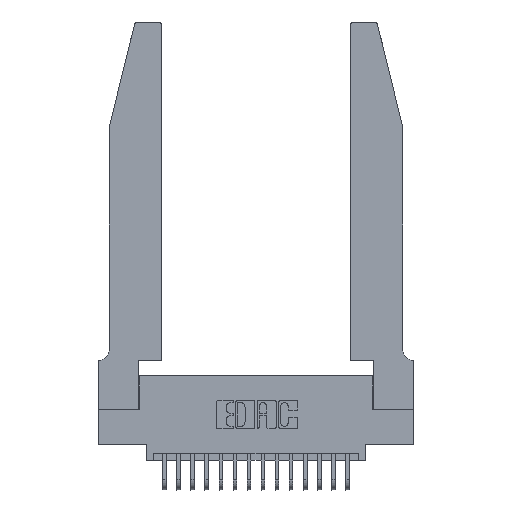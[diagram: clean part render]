
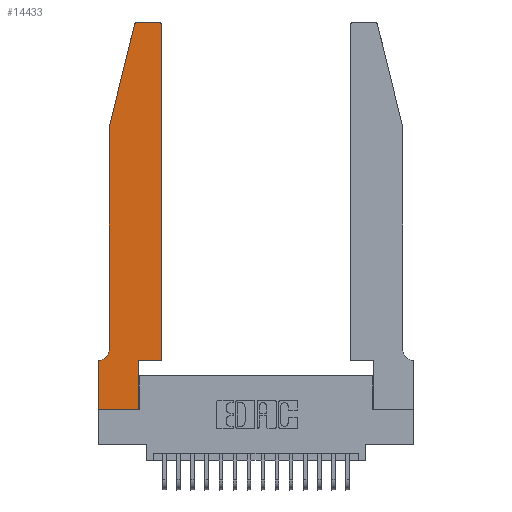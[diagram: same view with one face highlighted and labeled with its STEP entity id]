
A CAD part, top view. The second image highlights one B-rep face of the part: STEP entity #14433.
In plain terms, the highlighted planar face has unit normal (0, 0, 1).
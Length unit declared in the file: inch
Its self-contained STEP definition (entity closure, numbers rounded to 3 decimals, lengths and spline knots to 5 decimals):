
#6 = ORIENTED_EDGE ( 'NONE', *, *, #21173, .T. ) ;
#166 = VERTEX_POINT ( 'NONE', #15257 ) ;
#196 = EDGE_CURVE ( 'NONE', #13530, #4539, #17031, .T. ) ;
#664 = EDGE_CURVE ( 'NONE', #4786, #18224, #4362, .T. ) ;
#1320 = ORIENTED_EDGE ( 'NONE', *, *, #18303, .T. ) ;
#1442 = DIRECTION ( 'NONE',  ( 0., 1., 0. ) ) ;
#1481 = EDGE_CURVE ( 'NONE', #16555, #20800, #13324, .T. ) ;
#1889 = VERTEX_POINT ( 'NONE', #13498 ) ;
#1890 = LINE ( 'NONE', #8039, #14753 ) ;
#2274 = CARTESIAN_POINT ( 'NONE',  ( 0.0755, 2., 0.37 ) ) ;
#2402 = CARTESIAN_POINT ( 'NONE',  ( 0.4505, 0.35, 0.37 ) ) ;
#2846 = VECTOR ( 'NONE', #16586, 39.37008 ) ;
#3107 = AXIS2_PLACEMENT_3D ( 'NONE', #10799, #10655, #14158 ) ;
#3645 = CARTESIAN_POINT ( 'NONE',  ( 0.284, 2.72, 0.37 ) ) ;
#4362 = LINE ( 'NONE', #14949, #2846 ) ;
#4539 = VERTEX_POINT ( 'NONE', #11368 ) ;
#4607 = ORIENTED_EDGE ( 'NONE', *, *, #1481, .T. ) ;
#4786 = VERTEX_POINT ( 'NONE', #20607 ) ;
#4927 = CIRCLE ( 'NONE', #15768, 0.03 ) ;
#5079 = AXIS2_PLACEMENT_3D ( 'NONE', #3645, #16730, #18179 ) ;
#5161 = LINE ( 'NONE', #2402, #12854 ) ;
#5383 = DIRECTION ( 'NONE',  ( -1., 0., 0. ) ) ;
#5917 = EDGE_LOOP ( 'NONE', ( #13122, #15151, #10997, #10688, #4607, #13922, #11732, #10229, #1320, #17083, #6, #9298 ) ) ;
#5925 = CARTESIAN_POINT ( 'NONE',  ( 0.4505, 0.35, 0.37 ) ) ;
#6440 = VECTOR ( 'NONE', #19181, 39.37008 ) ;
#6522 = LINE ( 'NONE', #5925, #12433 ) ;
#6703 = VECTOR ( 'NONE', #5383, 39.37008 ) ;
#7192 = DIRECTION ( 'NONE',  ( 0., 1., 0. ) ) ;
#7670 = CARTESIAN_POINT ( 'NONE',  ( 0.4205, 2.75, 0.37 ) ) ;
#7751 = EDGE_CURVE ( 'NONE', #9254, #16555, #1890, .T. ) ;
#7994 = CARTESIAN_POINT ( 'NONE',  ( 0., 0.35, 0.37 ) ) ;
#8039 = CARTESIAN_POINT ( 'NONE',  ( 0.0755, 2., 0.37 ) ) ;
#8050 = FACE_OUTER_BOUND ( 'NONE', #5917, .T. ) ;
#8185 = VERTEX_POINT ( 'NONE', #14021 ) ;
#8205 = PLANE ( 'NONE',  #20137 ) ;
#9013 = DIRECTION ( 'NONE',  ( 1., 0., 0. ) ) ;
#9200 = CARTESIAN_POINT ( 'NONE',  ( 0., 0.35, 0.37 ) ) ;
#9254 = VERTEX_POINT ( 'NONE', #2274 ) ;
#9298 = ORIENTED_EDGE ( 'NONE', *, *, #19952, .T. ) ;
#9540 = CARTESIAN_POINT ( 'NONE',  ( 0., 0., 0.37 ) ) ;
#9683 = LINE ( 'NONE', #9540, #13815 ) ;
#10229 = ORIENTED_EDGE ( 'NONE', *, *, #664, .T. ) ;
#10256 = CARTESIAN_POINT ( 'NONE',  ( 0.0755, 0.42, 0.37 ) ) ;
#10655 = DIRECTION ( 'NONE',  ( 0., 0., -1. ) ) ;
#10688 = ORIENTED_EDGE ( 'NONE', *, *, #7751, .T. ) ;
#10695 = CARTESIAN_POINT ( 'NONE',  ( 0.0755, 2., 0.37 ) ) ;
#10799 = CARTESIAN_POINT ( 'NONE',  ( 0.0055, 0.42, 0.37 ) ) ;
#10997 = ORIENTED_EDGE ( 'NONE', *, *, #16225, .T. ) ;
#11257 = CARTESIAN_POINT ( 'NONE',  ( 0.2865, 0.35, 0.37 ) ) ;
#11366 = DIRECTION ( 'NONE',  ( 0., 0., 1. ) ) ;
#11368 = CARTESIAN_POINT ( 'NONE',  ( 0.284, 2.75, 0.37 ) ) ;
#11428 = DIRECTION ( 'NONE',  ( 1., 0., 0. ) ) ;
#11732 = ORIENTED_EDGE ( 'NONE', *, *, #18145, .T. ) ;
#11772 = VERTEX_POINT ( 'NONE', #9200 ) ;
#12190 = CARTESIAN_POINT ( 'NONE',  ( 0.2605, 2.75, 0.37 ) ) ;
#12340 = CARTESIAN_POINT ( 'NONE',  ( 0.4505, 0.35, 0.37 ) ) ;
#12433 = VECTOR ( 'NONE', #14223, 39.37008 ) ;
#12854 = VECTOR ( 'NONE', #7192, 39.37008 ) ;
#13122 = ORIENTED_EDGE ( 'NONE', *, *, #196, .T. ) ;
#13324 = CIRCLE ( 'NONE', #3107, 0.07 ) ;
#13498 = CARTESIAN_POINT ( 'NONE',  ( 0.4505, 2.72, 0.37 ) ) ;
#13530 = VERTEX_POINT ( 'NONE', #7670 ) ;
#13815 = VECTOR ( 'NONE', #14551, 39.37008 ) ;
#13922 = ORIENTED_EDGE ( 'NONE', *, *, #15502, .T. ) ;
#14021 = CARTESIAN_POINT ( 'NONE',  ( 0.2865, 0.35, 0.37 ) ) ;
#14158 = DIRECTION ( 'NONE',  ( -1., 0., 0. ) ) ;
#14223 = DIRECTION ( 'NONE',  ( 1., 0., 0. ) ) ;
#14261 = EDGE_CURVE ( 'NONE', #8185, #18666, #6522, .T. ) ;
#14384 = DIRECTION ( 'NONE',  ( -1., 0., 0. ) ) ;
#14433 = ADVANCED_FACE ( 'NONE', ( #8050 ), #8205, .T. ) ;
#14469 = VECTOR ( 'NONE', #14384, 39.37008 ) ;
#14537 = EDGE_CURVE ( 'NONE', #4539, #166, #19425, .T. ) ;
#14551 = DIRECTION ( 'NONE',  ( 0., -1., 0. ) ) ;
#14753 = VECTOR ( 'NONE', #21311, 39.37008 ) ;
#14872 = VECTOR ( 'NONE', #1442, 39.37008 ) ;
#14949 = CARTESIAN_POINT ( 'NONE',  ( 0., 0., 0.37 ) ) ;
#15151 = ORIENTED_EDGE ( 'NONE', *, *, #14537, .T. ) ;
#15257 = CARTESIAN_POINT ( 'NONE',  ( 0.25487, 2.72718, 0.37 ) ) ;
#15502 = EDGE_CURVE ( 'NONE', #20800, #11772, #20160, .T. ) ;
#15768 = AXIS2_PLACEMENT_3D ( 'NONE', #18935, #19153, #9013 ) ;
#16225 = EDGE_CURVE ( 'NONE', #166, #9254, #21124, .T. ) ;
#16555 = VERTEX_POINT ( 'NONE', #10256 ) ;
#16586 = DIRECTION ( 'NONE',  ( 1., 0., 0. ) ) ;
#16730 = DIRECTION ( 'NONE',  ( 0., 0., 1. ) ) ;
#17031 = LINE ( 'NONE', #12190, #6703 ) ;
#17083 = ORIENTED_EDGE ( 'NONE', *, *, #14261, .T. ) ;
#17579 = CARTESIAN_POINT ( 'NONE',  ( 0.2865, 0., 0.37 ) ) ;
#18145 = EDGE_CURVE ( 'NONE', #11772, #4786, #9683, .T. ) ;
#18179 = DIRECTION ( 'NONE',  ( 1., 0., 0. ) ) ;
#18224 = VERTEX_POINT ( 'NONE', #17579 ) ;
#18303 = EDGE_CURVE ( 'NONE', #18224, #8185, #19015, .T. ) ;
#18666 = VERTEX_POINT ( 'NONE', #12340 ) ;
#18935 = CARTESIAN_POINT ( 'NONE',  ( 0.4205, 2.72, 0.37 ) ) ;
#19015 = LINE ( 'NONE', #11257, #14872 ) ;
#19153 = DIRECTION ( 'NONE',  ( 0., 0., 1. ) ) ;
#19181 = DIRECTION ( 'NONE',  ( -0.239, -0.971, 0. ) ) ;
#19380 = CARTESIAN_POINT ( 'NONE',  ( 0.0755, 0.35, 0.37 ) ) ;
#19425 = CIRCLE ( 'NONE', #5079, 0.03 ) ;
#19624 = CARTESIAN_POINT ( 'NONE',  ( 0.0055, 0.35, 0.37 ) ) ;
#19952 = EDGE_CURVE ( 'NONE', #1889, #13530, #4927, .T. ) ;
#20137 = AXIS2_PLACEMENT_3D ( 'NONE', #7994, #11366, #11428 ) ;
#20160 = LINE ( 'NONE', #19380, #14469 ) ;
#20607 = CARTESIAN_POINT ( 'NONE',  ( 0., 0., 0.37 ) ) ;
#20800 = VERTEX_POINT ( 'NONE', #19624 ) ;
#21124 = LINE ( 'NONE', #10695, #6440 ) ;
#21173 = EDGE_CURVE ( 'NONE', #18666, #1889, #5161, .T. ) ;
#21311 = DIRECTION ( 'NONE',  ( 0., -1., 0. ) ) ;
